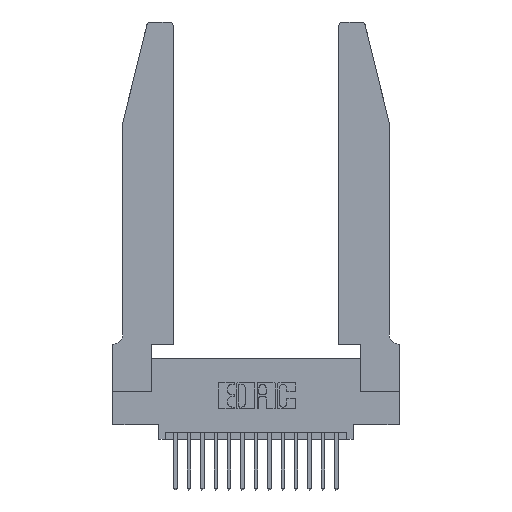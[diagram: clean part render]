
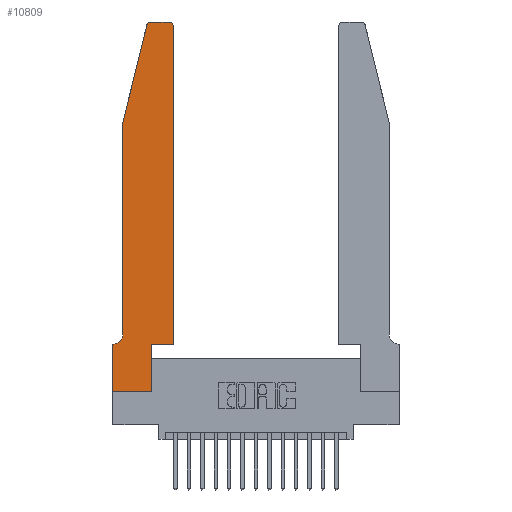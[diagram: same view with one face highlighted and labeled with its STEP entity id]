
A CAD part, top view. The second image highlights one B-rep face of the part: STEP entity #10809.
In plain terms, the highlighted planar face has unit normal (0, 0, 1).
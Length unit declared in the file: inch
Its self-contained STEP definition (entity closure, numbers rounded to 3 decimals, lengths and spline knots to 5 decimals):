
#86 = LINE ( 'NONE', #13681, #13843 ) ;
#94 = VERTEX_POINT ( 'NONE', #3468 ) ;
#212 = CARTESIAN_POINT ( 'NONE',  ( 0.2865, 0.35, 0.37 ) ) ;
#317 = CARTESIAN_POINT ( 'NONE',  ( 0.25487, 2.72718, 0.37 ) ) ;
#429 = VECTOR ( 'NONE', #9445, 39.37008 ) ;
#502 = CIRCLE ( 'NONE', #2411, 0.07 ) ;
#577 = CARTESIAN_POINT ( 'NONE',  ( 0.4505, 0.35, 0.37 ) ) ;
#688 = VERTEX_POINT ( 'NONE', #6293 ) ;
#706 = VERTEX_POINT ( 'NONE', #212 ) ;
#952 = EDGE_CURVE ( 'NONE', #9300, #18811, #14167, .T. ) ;
#1115 = VECTOR ( 'NONE', #16915, 39.37008 ) ;
#1359 = CARTESIAN_POINT ( 'NONE',  ( 0.284, 2.72, 0.37 ) ) ;
#1898 = DIRECTION ( 'NONE',  ( 0., -1., 0. ) ) ;
#2023 = EDGE_LOOP ( 'NONE', ( #16790, #8045, #15103, #15679, #6572, #12189, #3413, #12678, #8553, #3675, #13335, #11900 ) ) ;
#2094 = VERTEX_POINT ( 'NONE', #12372 ) ;
#2411 = AXIS2_PLACEMENT_3D ( 'NONE', #11339, #8461, #18729 ) ;
#2654 = CARTESIAN_POINT ( 'NONE',  ( 0.4505, 0.35, 0.37 ) ) ;
#2980 = CARTESIAN_POINT ( 'NONE',  ( 0.0755, 2., 0.37 ) ) ;
#3191 = LINE ( 'NONE', #18616, #1115 ) ;
#3413 = ORIENTED_EDGE ( 'NONE', *, *, #4447, .T. ) ;
#3468 = CARTESIAN_POINT ( 'NONE',  ( 0., 0.35, 0.37 ) ) ;
#3547 = CARTESIAN_POINT ( 'NONE',  ( 0.0755, 2., 0.37 ) ) ;
#3649 = VERTEX_POINT ( 'NONE', #16663 ) ;
#3675 = ORIENTED_EDGE ( 'NONE', *, *, #11181, .T. ) ;
#3996 = DIRECTION ( 'NONE',  ( 0., 0., 1. ) ) ;
#4447 = EDGE_CURVE ( 'NONE', #94, #3649, #3191, .T. ) ;
#4591 = VERTEX_POINT ( 'NONE', #317 ) ;
#4864 = DIRECTION ( 'NONE',  ( 1., 0., 0. ) ) ;
#5231 = EDGE_CURVE ( 'NONE', #688, #706, #10270, .T. ) ;
#5306 = DIRECTION ( 'NONE',  ( -1., 0., 0. ) ) ;
#5504 = CARTESIAN_POINT ( 'NONE',  ( 0., 0.35, 0.37 ) ) ;
#6069 = VERTEX_POINT ( 'NONE', #17406 ) ;
#6293 = CARTESIAN_POINT ( 'NONE',  ( 0.2865, 0., 0.37 ) ) ;
#6354 = VERTEX_POINT ( 'NONE', #2980 ) ;
#6444 = EDGE_CURVE ( 'NONE', #4591, #6354, #18939, .T. ) ;
#6542 = CARTESIAN_POINT ( 'NONE',  ( 0.2605, 2.75, 0.37 ) ) ;
#6572 = ORIENTED_EDGE ( 'NONE', *, *, #10760, .T. ) ;
#7015 = DIRECTION ( 'NONE',  ( 1., 0., 0. ) ) ;
#7121 = VERTEX_POINT ( 'NONE', #2654 ) ;
#7303 = LINE ( 'NONE', #6542, #429 ) ;
#7327 = DIRECTION ( 'NONE',  ( 1., 0., 0. ) ) ;
#7639 = LINE ( 'NONE', #12605, #18872 ) ;
#8045 = ORIENTED_EDGE ( 'NONE', *, *, #12731, .T. ) ;
#8076 = VERTEX_POINT ( 'NONE', #16088 ) ;
#8181 = VECTOR ( 'NONE', #16841, 39.37008 ) ;
#8192 = EDGE_CURVE ( 'NONE', #6069, #94, #7639, .T. ) ;
#8461 = DIRECTION ( 'NONE',  ( 0., 0., -1. ) ) ;
#8475 = CARTESIAN_POINT ( 'NONE',  ( 0., 0., 0.37 ) ) ;
#8517 = VECTOR ( 'NONE', #4864, 39.37008 ) ;
#8553 = ORIENTED_EDGE ( 'NONE', *, *, #5231, .T. ) ;
#9000 = CARTESIAN_POINT ( 'NONE',  ( 0.4505, 2.72, 0.37 ) ) ;
#9236 = FACE_OUTER_BOUND ( 'NONE', #2023, .T. ) ;
#9300 = VERTEX_POINT ( 'NONE', #9000 ) ;
#9445 = DIRECTION ( 'NONE',  ( -1., 0., 0. ) ) ;
#9615 = AXIS2_PLACEMENT_3D ( 'NONE', #16920, #3996, #14217 ) ;
#10007 = PLANE ( 'NONE',  #12356 ) ;
#10270 = LINE ( 'NONE', #11151, #13221 ) ;
#10400 = EDGE_CURVE ( 'NONE', #7121, #9300, #12881, .T. ) ;
#10760 = EDGE_CURVE ( 'NONE', #2094, #6069, #502, .T. ) ;
#10809 = ADVANCED_FACE ( 'NONE', ( #9236 ), #10007, .T. ) ;
#11151 = CARTESIAN_POINT ( 'NONE',  ( 0.2865, 0.35, 0.37 ) ) ;
#11181 = EDGE_CURVE ( 'NONE', #706, #7121, #16813, .T. ) ;
#11269 = DIRECTION ( 'NONE',  ( 0., 1., 0. ) ) ;
#11339 = CARTESIAN_POINT ( 'NONE',  ( 0.0055, 0.42, 0.37 ) ) ;
#11900 = ORIENTED_EDGE ( 'NONE', *, *, #952, .T. ) ;
#12189 = ORIENTED_EDGE ( 'NONE', *, *, #8192, .T. ) ;
#12257 = EDGE_CURVE ( 'NONE', #3649, #688, #15797, .T. ) ;
#12356 = AXIS2_PLACEMENT_3D ( 'NONE', #5504, #15821, #14328 ) ;
#12372 = CARTESIAN_POINT ( 'NONE',  ( 0.0755, 0.42, 0.37 ) ) ;
#12429 = DIRECTION ( 'NONE',  ( 0., 1., 0. ) ) ;
#12451 = EDGE_CURVE ( 'NONE', #18811, #8076, #7303, .T. ) ;
#12605 = CARTESIAN_POINT ( 'NONE',  ( 0.0755, 0.35, 0.37 ) ) ;
#12678 = ORIENTED_EDGE ( 'NONE', *, *, #12257, .T. ) ;
#12731 = EDGE_CURVE ( 'NONE', #8076, #4591, #17654, .T. ) ;
#12881 = LINE ( 'NONE', #577, #15654 ) ;
#13221 = VECTOR ( 'NONE', #11269, 39.37008 ) ;
#13335 = ORIENTED_EDGE ( 'NONE', *, *, #10400, .T. ) ;
#13681 = CARTESIAN_POINT ( 'NONE',  ( 0.0755, 2., 0.37 ) ) ;
#13843 = VECTOR ( 'NONE', #1898, 39.37008 ) ;
#14167 = CIRCLE ( 'NONE', #9615, 0.03 ) ;
#14217 = DIRECTION ( 'NONE',  ( 1., 0., 0. ) ) ;
#14328 = DIRECTION ( 'NONE',  ( 1., 0., 0. ) ) ;
#14477 = DIRECTION ( 'NONE',  ( 0., 0., 1. ) ) ;
#15103 = ORIENTED_EDGE ( 'NONE', *, *, #6444, .T. ) ;
#15654 = VECTOR ( 'NONE', #12429, 39.37008 ) ;
#15679 = ORIENTED_EDGE ( 'NONE', *, *, #16711, .T. ) ;
#15797 = LINE ( 'NONE', #8475, #17414 ) ;
#15821 = DIRECTION ( 'NONE',  ( 0., 0., 1. ) ) ;
#16088 = CARTESIAN_POINT ( 'NONE',  ( 0.284, 2.75, 0.37 ) ) ;
#16215 = AXIS2_PLACEMENT_3D ( 'NONE', #1359, #14477, #7327 ) ;
#16663 = CARTESIAN_POINT ( 'NONE',  ( 0., 0., 0.37 ) ) ;
#16711 = EDGE_CURVE ( 'NONE', #6354, #2094, #86, .T. ) ;
#16790 = ORIENTED_EDGE ( 'NONE', *, *, #12451, .T. ) ;
#16813 = LINE ( 'NONE', #18098, #8517 ) ;
#16841 = DIRECTION ( 'NONE',  ( -0.239, -0.971, 0. ) ) ;
#16915 = DIRECTION ( 'NONE',  ( 0., -1., 0. ) ) ;
#16920 = CARTESIAN_POINT ( 'NONE',  ( 0.4205, 2.72, 0.37 ) ) ;
#17406 = CARTESIAN_POINT ( 'NONE',  ( 0.0055, 0.35, 0.37 ) ) ;
#17414 = VECTOR ( 'NONE', #7015, 39.37008 ) ;
#17525 = CARTESIAN_POINT ( 'NONE',  ( 0.4205, 2.75, 0.37 ) ) ;
#17654 = CIRCLE ( 'NONE', #16215, 0.03 ) ;
#18098 = CARTESIAN_POINT ( 'NONE',  ( 0.4505, 0.35, 0.37 ) ) ;
#18616 = CARTESIAN_POINT ( 'NONE',  ( 0., 0., 0.37 ) ) ;
#18729 = DIRECTION ( 'NONE',  ( -1., 0., 0. ) ) ;
#18811 = VERTEX_POINT ( 'NONE', #17525 ) ;
#18872 = VECTOR ( 'NONE', #5306, 39.37008 ) ;
#18939 = LINE ( 'NONE', #3547, #8181 ) ;
